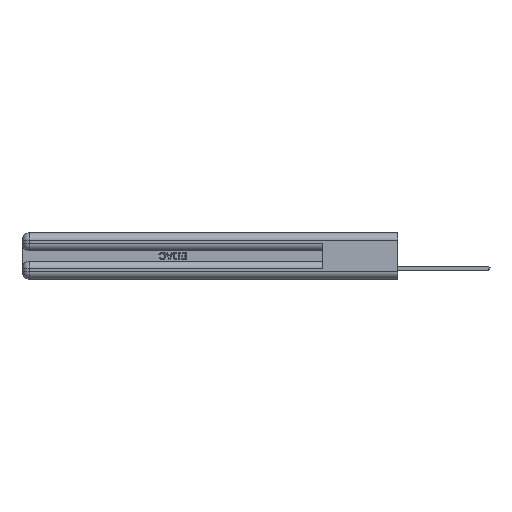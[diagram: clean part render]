
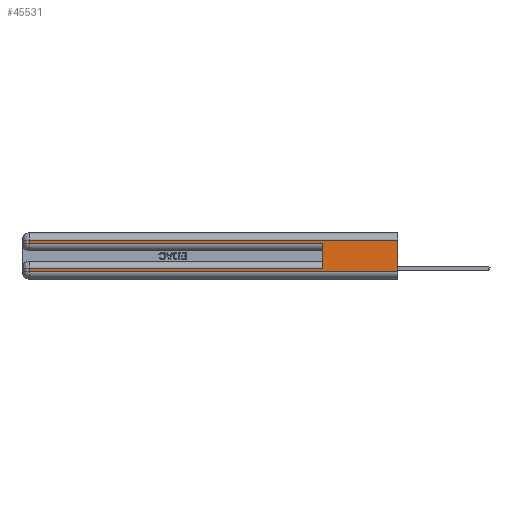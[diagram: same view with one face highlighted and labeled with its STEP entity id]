
A CAD part, left-side view. The second image highlights one B-rep face of the part: STEP entity #45531.
In plain terms, the highlighted planar face has unit normal (-1, 0, 0).
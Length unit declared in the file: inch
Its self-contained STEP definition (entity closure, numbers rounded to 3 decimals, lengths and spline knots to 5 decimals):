
#1829 = LINE ( 'NONE', #43980, #39958 ) ;
#1889 = AXIS2_PLACEMENT_3D ( 'NONE', #35182, #14056, #3248 ) ;
#2870 = EDGE_CURVE ( 'NONE', #13826, #8417, #17953, .T. ) ;
#2874 = CARTESIAN_POINT ( 'NONE',  ( 0., 2.94, 0.06 ) ) ;
#3248 = DIRECTION ( 'NONE',  ( 0., 0., -1. ) ) ;
#4129 = CARTESIAN_POINT ( 'NONE',  ( 0., 0., 0.285 ) ) ;
#4237 = EDGE_CURVE ( 'NONE', #25828, #41509, #11492, .T. ) ;
#4567 = VECTOR ( 'NONE', #8600, 39.37008 ) ;
#5642 = VERTEX_POINT ( 'NONE', #2874 ) ;
#8417 = VERTEX_POINT ( 'NONE', #38715 ) ;
#8600 = DIRECTION ( 'NONE',  ( 0., -1., 0. ) ) ;
#8821 = VECTOR ( 'NONE', #20164, 39.37008 ) ;
#11448 = CARTESIAN_POINT ( 'NONE',  ( 0., 0.6, 0.145 ) ) ;
#11492 = LINE ( 'NONE', #4129, #4567 ) ;
#11661 = CARTESIAN_POINT ( 'NONE',  ( 0., 0., 0.31 ) ) ;
#12181 = DIRECTION ( 'NONE',  ( 0., 0., -1. ) ) ;
#12694 = CARTESIAN_POINT ( 'NONE',  ( 0., 2.94, 0.31 ) ) ;
#12770 = CARTESIAN_POINT ( 'NONE',  ( 0., 2.94, 0.37 ) ) ;
#13751 = EDGE_CURVE ( 'NONE', #23027, #5642, #44059, .T. ) ;
#13826 = VERTEX_POINT ( 'NONE', #25341 ) ;
#14029 = VECTOR ( 'NONE', #19230, 39.37008 ) ;
#14056 = DIRECTION ( 'NONE',  ( 1., 0., 0. ) ) ;
#14106 = VECTOR ( 'NONE', #12181, 39.37008 ) ;
#14466 = EDGE_CURVE ( 'NONE', #29686, #25828, #42887, .T. ) ;
#15965 = EDGE_CURVE ( 'NONE', #5642, #8417, #43471, .T. ) ;
#16640 = EDGE_CURVE ( 'NONE', #43370, #41509, #20959, .T. ) ;
#17268 = EDGE_CURVE ( 'NONE', #43370, #23027, #1829, .T. ) ;
#17490 = LINE ( 'NONE', #11661, #14029 ) ;
#17953 = LINE ( 'NONE', #40385, #41071 ) ;
#18052 = DIRECTION ( 'NONE',  ( 0., -1., 0. ) ) ;
#19158 = ORIENTED_EDGE ( 'NONE', *, *, #14466, .T. ) ;
#19230 = DIRECTION ( 'NONE',  ( 0., 1., 0. ) ) ;
#19994 = CARTESIAN_POINT ( 'NONE',  ( 0., 0.6, 0.085 ) ) ;
#20164 = DIRECTION ( 'NONE',  ( 0., 0., -1. ) ) ;
#20959 = LINE ( 'NONE', #11448, #24982 ) ;
#21457 = PLANE ( 'NONE',  #1889 ) ;
#21587 = ORIENTED_EDGE ( 'NONE', *, *, #23326, .T. ) ;
#22410 = FACE_OUTER_BOUND ( 'NONE', #33608, .T. ) ;
#22942 = CARTESIAN_POINT ( 'NONE',  ( 0., 2.94, 0.37 ) ) ;
#23027 = VERTEX_POINT ( 'NONE', #34302 ) ;
#23097 = ORIENTED_EDGE ( 'NONE', *, *, #4237, .T. ) ;
#23326 = EDGE_CURVE ( 'NONE', #13826, #29686, #17490, .T. ) ;
#24982 = VECTOR ( 'NONE', #25269, 39.37008 ) ;
#25269 = DIRECTION ( 'NONE',  ( 0., 0., 1. ) ) ;
#25341 = CARTESIAN_POINT ( 'NONE',  ( 0., 0., 0.31 ) ) ;
#25828 = VERTEX_POINT ( 'NONE', #38522 ) ;
#29686 = VERTEX_POINT ( 'NONE', #12694 ) ;
#33278 = DIRECTION ( 'NONE',  ( 0., 0., -1. ) ) ;
#33354 = DIRECTION ( 'NONE',  ( 0., 1., 0. ) ) ;
#33608 = EDGE_LOOP ( 'NONE', ( #38205, #21587, #19158, #23097, #35386, #38748, #41012, #36947 ) ) ;
#34302 = CARTESIAN_POINT ( 'NONE',  ( 0., 2.94, 0.085 ) ) ;
#35182 = CARTESIAN_POINT ( 'NONE',  ( 0., 0., 0.37 ) ) ;
#35386 = ORIENTED_EDGE ( 'NONE', *, *, #16640, .F. ) ;
#36947 = ORIENTED_EDGE ( 'NONE', *, *, #15965, .T. ) ;
#38205 = ORIENTED_EDGE ( 'NONE', *, *, #2870, .F. ) ;
#38329 = VECTOR ( 'NONE', #18052, 39.37008 ) ;
#38522 = CARTESIAN_POINT ( 'NONE',  ( 0., 2.94, 0.285 ) ) ;
#38715 = CARTESIAN_POINT ( 'NONE',  ( 0., 0., 0.06 ) ) ;
#38748 = ORIENTED_EDGE ( 'NONE', *, *, #17268, .T. ) ;
#39958 = VECTOR ( 'NONE', #33354, 39.37008 ) ;
#40385 = CARTESIAN_POINT ( 'NONE',  ( 0., 0., 0.37 ) ) ;
#41012 = ORIENTED_EDGE ( 'NONE', *, *, #13751, .T. ) ;
#41071 = VECTOR ( 'NONE', #33278, 39.37008 ) ;
#41509 = VERTEX_POINT ( 'NONE', #44487 ) ;
#42887 = LINE ( 'NONE', #12770, #8821 ) ;
#43370 = VERTEX_POINT ( 'NONE', #19994 ) ;
#43471 = LINE ( 'NONE', #47375, #38329 ) ;
#43980 = CARTESIAN_POINT ( 'NONE',  ( 0., 0., 0.085 ) ) ;
#44059 = LINE ( 'NONE', #22942, #14106 ) ;
#44487 = CARTESIAN_POINT ( 'NONE',  ( 0., 0.6, 0.285 ) ) ;
#45531 = ADVANCED_FACE ( 'NONE', ( #22410 ), #21457, .F. ) ;
#47375 = CARTESIAN_POINT ( 'NONE',  ( 0., 0., 0.06 ) ) ;
